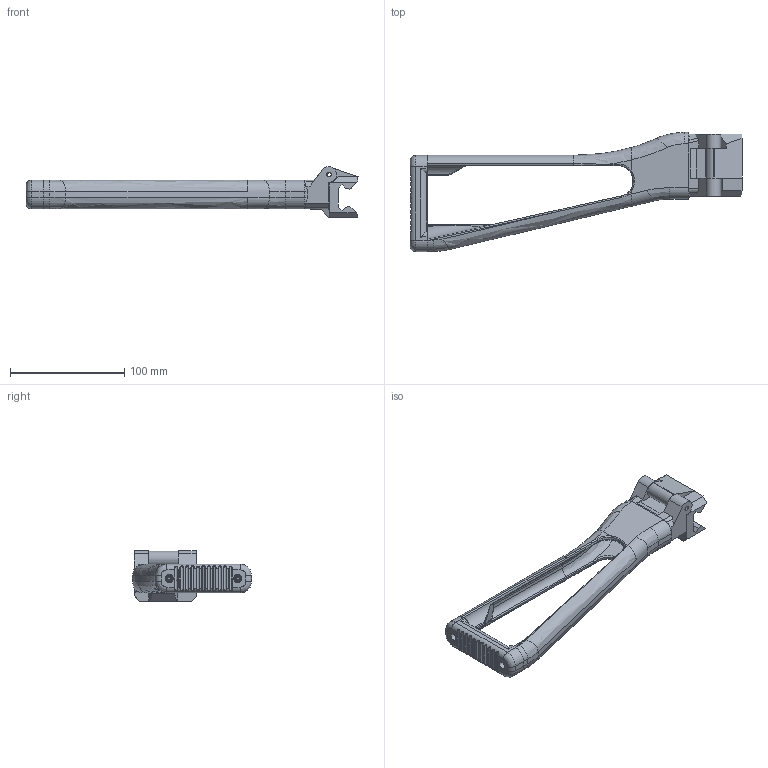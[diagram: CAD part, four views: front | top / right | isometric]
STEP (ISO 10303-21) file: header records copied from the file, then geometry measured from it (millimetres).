
FILE_DESCRIPTION(/* description */ (''),/* implementation_level */ '2;1');
FILE_NAME(/* author */ (''),/* organization */ (''),/* preprocessor_version */ 'ST-DEVELOPER v15.2',/* originating_system */ 'Autodesk Translator Framework v2.0.0.5431',/* authorisation */ '');
FILE_SCHEMA (('AUTOMOTIVE_DESIGN { 1 0 10303 214 3 1 1 }'));
Length unit declared in the file: centimetre
Products named in the file (1): MOD 22X SCAR EDITION retract v2
Bounding box: 290.65 x 104.31 x 44.3 mm (x, y, z)
Volume: 186443.6 mm3; surface area: 66446.4 mm2
Topology: 4 solids, 4 shells, 406 faces, 1079 edges, 686 vertices
Faces by surface type: plane 140, cylinder 120, bspline 117, torus 16, cone 11, sphere 2
Full cylindrical faces by diameter (mm): 3 x1, 3.5 x2, 4 x3, 6.5 x2, 12.1 x1, 20.5 x1
Entity records: 17458 total; most frequent: CARTESIAN_POINT 7989, ORIENTED_EDGE 2116, DIRECTION 1765, EDGE_CURVE 1058, VERTEX_POINT 683, AXIS2_PLACEMENT_3D 647, LINE 471, VECTOR 471
